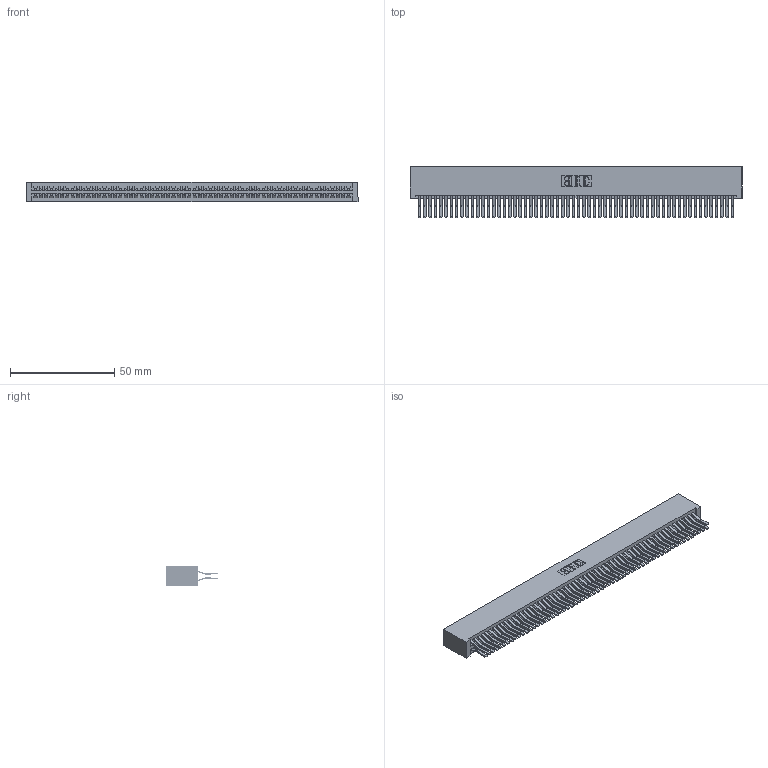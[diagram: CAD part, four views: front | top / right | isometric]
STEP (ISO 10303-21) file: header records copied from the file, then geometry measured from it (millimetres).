
FILE_DESCRIPTION (( 'STEP AP203' ), '1' );
FILE_NAME ('345-120-560-201.STEP', '2019-11-06T11:41:58', ( '' ), ( '' ), 'SwSTEP 2.0', 'SolidWorks 2016', '' );
FILE_SCHEMA (( 'CONFIG_CONTROL_DESIGN' ));
Length unit declared in the file: inch
Products named in the file (3): 345-120-560-201; 345-292-001_560 Tail; 345 Part_No Mounting Lugs
Assembly tree (121 placements, depth 2):
  345-120-560-201
    345 Part_No Mounting Lugs
    345-292-001_560 Tail  x120
Bounding box: 159 x 24.45 x 9.4 mm (x, y, z)
Volume: 17015.4 mm3; surface area: 27826.4 mm2
Topology: 121 solids, 121 shells, 6358 faces, 18917 edges, 12450 vertices
Faces by surface type: plane 4036, cylinder 2322
Entity records: 44465 total; most frequent: CARTESIAN_POINT 7436, ORIENTED_EDGE 7370, DIRECTION 6533, EDGE_CURVE 3685, VECTOR 3317, LINE 3317, VERTEX_POINT 2454, AXIS2_PLACEMENT_3D 1608
